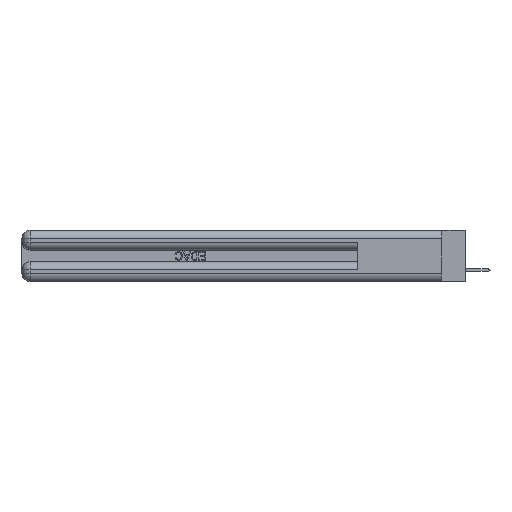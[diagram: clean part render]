
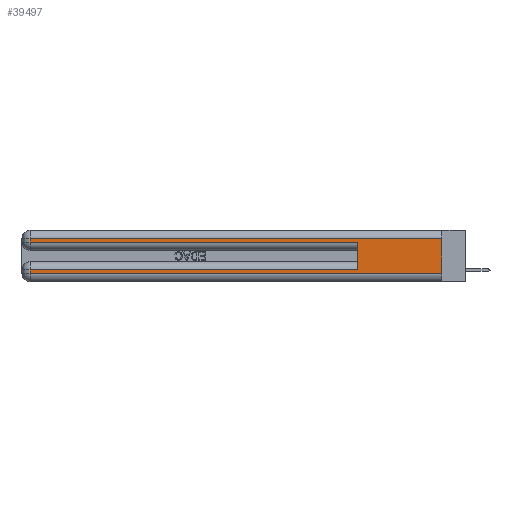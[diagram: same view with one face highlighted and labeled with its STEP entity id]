
A CAD part, left-side view. The second image highlights one B-rep face of the part: STEP entity #39497.
In plain terms, the highlighted planar face has unit normal (-1, 0, 0).
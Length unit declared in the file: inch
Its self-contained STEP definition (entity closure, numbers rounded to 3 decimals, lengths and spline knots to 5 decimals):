
#850 = ORIENTED_EDGE ( 'NONE', *, *, #32776, .T. ) ;
#949 = PLANE ( 'NONE',  #16507 ) ;
#1132 = DIRECTION ( 'NONE',  ( 1., 0., 0. ) ) ;
#1572 = CARTESIAN_POINT ( 'NONE',  ( 0., 2.94, 0.37 ) ) ;
#1623 = DIRECTION ( 'NONE',  ( 0., -1., 0. ) ) ;
#1827 = DIRECTION ( 'NONE',  ( 0., -1., 0. ) ) ;
#2429 = LINE ( 'NONE', #6662, #21743 ) ;
#2897 = VECTOR ( 'NONE', #1623, 39.37008 ) ;
#3081 = CARTESIAN_POINT ( 'NONE',  ( 0., 0.6, 0.145 ) ) ;
#4803 = EDGE_CURVE ( 'NONE', #6194, #39764, #35908, .T. ) ;
#6135 = LINE ( 'NONE', #13462, #43758 ) ;
#6194 = VERTEX_POINT ( 'NONE', #26381 ) ;
#6662 = CARTESIAN_POINT ( 'NONE',  ( 0., 2.94, 0.37 ) ) ;
#7330 = VERTEX_POINT ( 'NONE', #47955 ) ;
#7421 = ORIENTED_EDGE ( 'NONE', *, *, #28734, .F. ) ;
#7736 = EDGE_CURVE ( 'NONE', #39764, #7330, #2429, .T. ) ;
#12346 = CARTESIAN_POINT ( 'NONE',  ( 0., 0., 0.06 ) ) ;
#12768 = ORIENTED_EDGE ( 'NONE', *, *, #23283, .T. ) ;
#12984 = LINE ( 'NONE', #23281, #51870 ) ;
#13462 = CARTESIAN_POINT ( 'NONE',  ( 0., 0., 0.085 ) ) ;
#14574 = DIRECTION ( 'NONE',  ( 0., 1., 0. ) ) ;
#15655 = ORIENTED_EDGE ( 'NONE', *, *, #26108, .F. ) ;
#15844 = FACE_OUTER_BOUND ( 'NONE', #45275, .T. ) ;
#16507 = AXIS2_PLACEMENT_3D ( 'NONE', #32452, #1132, #16674 ) ;
#16674 = DIRECTION ( 'NONE',  ( 0., 0., -1. ) ) ;
#17741 = CARTESIAN_POINT ( 'NONE',  ( 0., 0.6, 0.085 ) ) ;
#18174 = EDGE_CURVE ( 'NONE', #7330, #32544, #39884, .T. ) ;
#18310 = VECTOR ( 'NONE', #29529, 39.37008 ) ;
#19127 = CARTESIAN_POINT ( 'NONE',  ( 0., 2.94, 0.06 ) ) ;
#19322 = VERTEX_POINT ( 'NONE', #17741 ) ;
#19507 = VECTOR ( 'NONE', #14574, 39.37008 ) ;
#20053 = CARTESIAN_POINT ( 'NONE',  ( 0., 2.94, 0.085 ) ) ;
#21743 = VECTOR ( 'NONE', #46207, 39.37008 ) ;
#22787 = ORIENTED_EDGE ( 'NONE', *, *, #7736, .T. ) ;
#23281 = CARTESIAN_POINT ( 'NONE',  ( 0., 0., 0.37 ) ) ;
#23283 = EDGE_CURVE ( 'NONE', #50692, #38694, #31515, .T. ) ;
#24673 = CARTESIAN_POINT ( 'NONE',  ( 0., 0., 0.285 ) ) ;
#24963 = CARTESIAN_POINT ( 'NONE',  ( 0., 0.6, 0.285 ) ) ;
#25125 = LINE ( 'NONE', #3081, #35890 ) ;
#26108 = EDGE_CURVE ( 'NONE', #6194, #43610, #12984, .T. ) ;
#26381 = CARTESIAN_POINT ( 'NONE',  ( 0., 0., 0.31 ) ) ;
#26444 = CARTESIAN_POINT ( 'NONE',  ( 0., 0., 0.31 ) ) ;
#28734 = EDGE_CURVE ( 'NONE', #19322, #32544, #25125, .T. ) ;
#29529 = DIRECTION ( 'NONE',  ( 0., 0., -1. ) ) ;
#29976 = EDGE_CURVE ( 'NONE', #38694, #43610, #30739, .T. ) ;
#30739 = LINE ( 'NONE', #45425, #48295 ) ;
#31515 = LINE ( 'NONE', #1572, #18310 ) ;
#32452 = CARTESIAN_POINT ( 'NONE',  ( 0., 0., 0.37 ) ) ;
#32544 = VERTEX_POINT ( 'NONE', #24963 ) ;
#32776 = EDGE_CURVE ( 'NONE', #19322, #50692, #6135, .T. ) ;
#34577 = CARTESIAN_POINT ( 'NONE',  ( 0., 2.94, 0.31 ) ) ;
#35890 = VECTOR ( 'NONE', #40011, 39.37008 ) ;
#35908 = LINE ( 'NONE', #26444, #19507 ) ;
#38694 = VERTEX_POINT ( 'NONE', #19127 ) ;
#39497 = ADVANCED_FACE ( 'NONE', ( #15844 ), #949, .F. ) ;
#39764 = VERTEX_POINT ( 'NONE', #34577 ) ;
#39798 = DIRECTION ( 'NONE',  ( 0., 0., -1. ) ) ;
#39884 = LINE ( 'NONE', #24673, #2897 ) ;
#40011 = DIRECTION ( 'NONE',  ( 0., 0., 1. ) ) ;
#41680 = DIRECTION ( 'NONE',  ( 0., 1., 0. ) ) ;
#43610 = VERTEX_POINT ( 'NONE', #12346 ) ;
#43758 = VECTOR ( 'NONE', #41680, 39.37008 ) ;
#45275 = EDGE_LOOP ( 'NONE', ( #15655, #46108, #22787, #46701, #7421, #850, #12768, #48619 ) ) ;
#45425 = CARTESIAN_POINT ( 'NONE',  ( 0., 0., 0.06 ) ) ;
#46108 = ORIENTED_EDGE ( 'NONE', *, *, #4803, .T. ) ;
#46207 = DIRECTION ( 'NONE',  ( 0., 0., -1. ) ) ;
#46701 = ORIENTED_EDGE ( 'NONE', *, *, #18174, .T. ) ;
#47955 = CARTESIAN_POINT ( 'NONE',  ( 0., 2.94, 0.285 ) ) ;
#48295 = VECTOR ( 'NONE', #1827, 39.37008 ) ;
#48619 = ORIENTED_EDGE ( 'NONE', *, *, #29976, .T. ) ;
#50692 = VERTEX_POINT ( 'NONE', #20053 ) ;
#51870 = VECTOR ( 'NONE', #39798, 39.37008 ) ;
